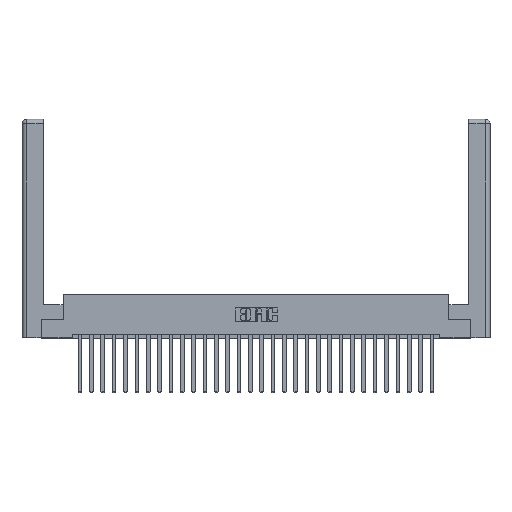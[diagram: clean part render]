
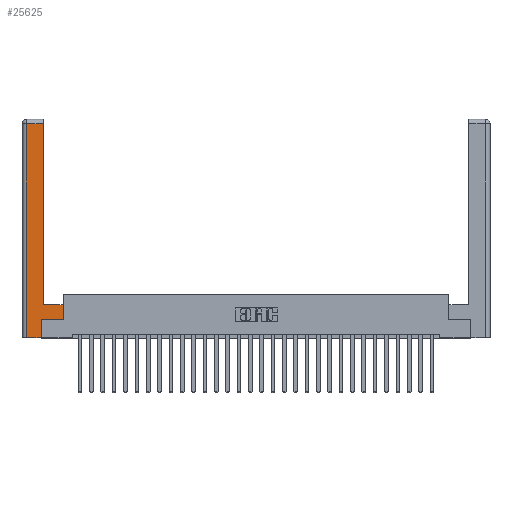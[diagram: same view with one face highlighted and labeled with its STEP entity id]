
A CAD part, top view. The second image highlights one B-rep face of the part: STEP entity #25625.
In plain terms, the highlighted planar face has unit normal (0, 0, 1).
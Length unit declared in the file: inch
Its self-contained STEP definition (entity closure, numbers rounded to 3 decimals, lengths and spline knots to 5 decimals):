
#86 = DIRECTION ( 'NONE',  ( 0., 0., -1. ) ) ;
#210 = DIRECTION ( 'NONE',  ( 0., 1., 0. ) ) ;
#362 = ORIENTED_EDGE ( 'NONE', *, *, #14323, .T. ) ;
#1255 = ORIENTED_EDGE ( 'NONE', *, *, #23349, .T. ) ;
#1410 = VECTOR ( 'NONE', #27893, 39.37008 ) ;
#2528 = PLANE ( 'NONE',  #13815 ) ;
#2586 = VECTOR ( 'NONE', #210, 39.37008 ) ;
#2737 = EDGE_CURVE ( 'NONE', #13041, #10808, #12235, .T. ) ;
#2995 = VERTEX_POINT ( 'NONE', #19556 ) ;
#3012 = CARTESIAN_POINT ( 'NONE',  ( 0.295, 0.45, 0. ) ) ;
#3072 = VERTEX_POINT ( 'NONE', #15523 ) ;
#3881 = VERTEX_POINT ( 'NONE', #21829 ) ;
#5200 = ORIENTED_EDGE ( 'NONE', *, *, #6844, .T. ) ;
#6844 = EDGE_CURVE ( 'NONE', #23521, #3881, #18529, .T. ) ;
#7327 = LINE ( 'NONE', #21566, #1410 ) ;
#7746 = DIRECTION ( 'NONE',  ( -1., 0., 0. ) ) ;
#7888 = DIRECTION ( 'NONE',  ( 1., 0., 0. ) ) ;
#8960 = VECTOR ( 'NONE', #17544, 39.37008 ) ;
#9180 = CARTESIAN_POINT ( 'NONE',  ( 0.0615, 2.94, 0. ) ) ;
#10040 = CARTESIAN_POINT ( 'NONE',  ( 0.0615, 2.94, 0. ) ) ;
#10808 = VERTEX_POINT ( 'NONE', #9180 ) ;
#11025 = CARTESIAN_POINT ( 'NONE',  ( 0., 0., 0. ) ) ;
#11264 = VECTOR ( 'NONE', #21476, 39.37008 ) ;
#12235 = LINE ( 'NONE', #10040, #13627 ) ;
#12933 = LINE ( 'NONE', #13460, #2586 ) ;
#12997 = EDGE_CURVE ( 'NONE', #22646, #2995, #14081, .T. ) ;
#13041 = VERTEX_POINT ( 'NONE', #15260 ) ;
#13141 = ORIENTED_EDGE ( 'NONE', *, *, #19222, .T. ) ;
#13460 = CARTESIAN_POINT ( 'NONE',  ( 0.565, 0.45, 0. ) ) ;
#13627 = VECTOR ( 'NONE', #23264, 39.37008 ) ;
#13815 = AXIS2_PLACEMENT_3D ( 'NONE', #11025, #86, #24082 ) ;
#14081 = LINE ( 'NONE', #3012, #23662 ) ;
#14323 = EDGE_CURVE ( 'NONE', #10808, #23521, #18787, .T. ) ;
#14706 = LINE ( 'NONE', #23963, #22586 ) ;
#14708 = ORIENTED_EDGE ( 'NONE', *, *, #16582, .T. ) ;
#15260 = CARTESIAN_POINT ( 'NONE',  ( 0.295, 2.94, 0. ) ) ;
#15523 = CARTESIAN_POINT ( 'NONE',  ( 0.565, 0.245, 0. ) ) ;
#16294 = CARTESIAN_POINT ( 'NONE',  ( 0.565, 0.45, 0. ) ) ;
#16582 = EDGE_CURVE ( 'NONE', #3072, #22646, #12933, .T. ) ;
#17544 = DIRECTION ( 'NONE',  ( 1., 0., 0. ) ) ;
#17720 = CARTESIAN_POINT ( 'NONE',  ( 0.0615, 0., 0. ) ) ;
#18529 = LINE ( 'NONE', #21849, #8960 ) ;
#18787 = LINE ( 'NONE', #21192, #11264 ) ;
#19222 = EDGE_CURVE ( 'NONE', #2995, #13041, #7327, .T. ) ;
#19414 = EDGE_LOOP ( 'NONE', ( #13141, #26007, #362, #5200, #1255, #26350, #14708, #24544 ) ) ;
#19556 = CARTESIAN_POINT ( 'NONE',  ( 0.295, 0.45, 0. ) ) ;
#19736 = FACE_OUTER_BOUND ( 'NONE', #19414, .T. ) ;
#19911 = CARTESIAN_POINT ( 'NONE',  ( 0.265, 0.245, 0. ) ) ;
#20583 = LINE ( 'NONE', #23512, #20936 ) ;
#20936 = VECTOR ( 'NONE', #7888, 39.37008 ) ;
#21192 = CARTESIAN_POINT ( 'NONE',  ( 0.0615, 0., 0. ) ) ;
#21476 = DIRECTION ( 'NONE',  ( 0., -1., 0. ) ) ;
#21566 = CARTESIAN_POINT ( 'NONE',  ( 0.295, 3., 0. ) ) ;
#21829 = CARTESIAN_POINT ( 'NONE',  ( 0.265, 0., 0. ) ) ;
#21849 = CARTESIAN_POINT ( 'NONE',  ( 0.265, 0., 0. ) ) ;
#22501 = EDGE_CURVE ( 'NONE', #26411, #3072, #20583, .T. ) ;
#22586 = VECTOR ( 'NONE', #24071, 39.37008 ) ;
#22646 = VERTEX_POINT ( 'NONE', #16294 ) ;
#23264 = DIRECTION ( 'NONE',  ( -1., 0., 0. ) ) ;
#23349 = EDGE_CURVE ( 'NONE', #3881, #26411, #14706, .T. ) ;
#23512 = CARTESIAN_POINT ( 'NONE',  ( 0.565, 0.245, 0. ) ) ;
#23521 = VERTEX_POINT ( 'NONE', #17720 ) ;
#23662 = VECTOR ( 'NONE', #7746, 39.37008 ) ;
#23963 = CARTESIAN_POINT ( 'NONE',  ( 0.265, 0.245, 0. ) ) ;
#24071 = DIRECTION ( 'NONE',  ( 0., 1., 0. ) ) ;
#24082 = DIRECTION ( 'NONE',  ( -1., 0., 0. ) ) ;
#24544 = ORIENTED_EDGE ( 'NONE', *, *, #12997, .T. ) ;
#25625 = ADVANCED_FACE ( 'NONE', ( #19736 ), #2528, .F. ) ;
#26007 = ORIENTED_EDGE ( 'NONE', *, *, #2737, .T. ) ;
#26350 = ORIENTED_EDGE ( 'NONE', *, *, #22501, .T. ) ;
#26411 = VERTEX_POINT ( 'NONE', #19911 ) ;
#27893 = DIRECTION ( 'NONE',  ( 0., 1., 0. ) ) ;
